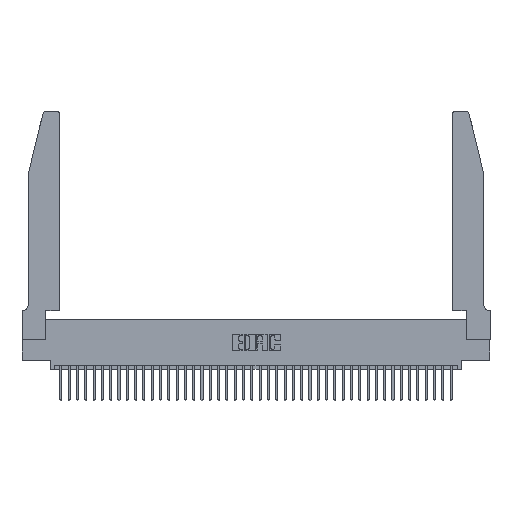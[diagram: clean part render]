
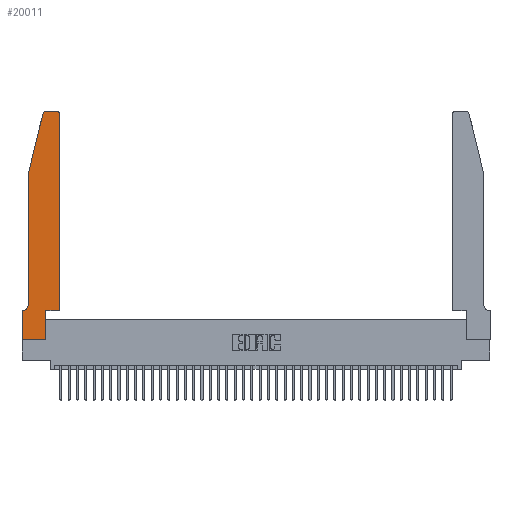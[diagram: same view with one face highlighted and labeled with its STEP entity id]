
A CAD part, top view. The second image highlights one B-rep face of the part: STEP entity #20011.
In plain terms, the highlighted planar face has unit normal (0, 0, 1).
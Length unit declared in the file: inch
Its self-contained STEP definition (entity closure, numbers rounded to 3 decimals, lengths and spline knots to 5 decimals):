
#8 = CARTESIAN_POINT ( 'NONE',  ( 0.0055, 0.42, 0.37 ) ) ;
#233 = VECTOR ( 'NONE', #17555, 39.37008 ) ;
#1323 = CARTESIAN_POINT ( 'NONE',  ( 0.4505, 0.35, 0.37 ) ) ;
#1931 = ORIENTED_EDGE ( 'NONE', *, *, #31756, .T. ) ;
#2160 = EDGE_CURVE ( 'NONE', #39411, #24685, #26172, .T. ) ;
#2168 = VECTOR ( 'NONE', #31009, 39.37008 ) ;
#2701 = VECTOR ( 'NONE', #29917, 39.37008 ) ;
#3124 = DIRECTION ( 'NONE',  ( 1., 0., 0. ) ) ;
#3176 = DIRECTION ( 'NONE',  ( 0., 0., 1. ) ) ;
#3357 = DIRECTION ( 'NONE',  ( -1., 0., 0. ) ) ;
#3690 = VERTEX_POINT ( 'NONE', #20641 ) ;
#3731 = LINE ( 'NONE', #10664, #2701 ) ;
#3998 = ORIENTED_EDGE ( 'NONE', *, *, #31245, .T. ) ;
#4175 = EDGE_CURVE ( 'NONE', #24613, #6546, #34977, .T. ) ;
#4821 = DIRECTION ( 'NONE',  ( 0., -1., 0. ) ) ;
#5491 = CARTESIAN_POINT ( 'NONE',  ( 0.2605, 2.75, 0.37 ) ) ;
#6411 = DIRECTION ( 'NONE',  ( 0., 0., 1. ) ) ;
#6546 = VERTEX_POINT ( 'NONE', #38351 ) ;
#7314 = CARTESIAN_POINT ( 'NONE',  ( 0.25487, 2.72718, 0.37 ) ) ;
#8202 = FACE_OUTER_BOUND ( 'NONE', #25432, .T. ) ;
#8244 = LINE ( 'NONE', #36824, #33868 ) ;
#8453 = VERTEX_POINT ( 'NONE', #12499 ) ;
#8723 = VECTOR ( 'NONE', #19870, 39.37008 ) ;
#10162 = EDGE_CURVE ( 'NONE', #8453, #3690, #25823, .T. ) ;
#10664 = CARTESIAN_POINT ( 'NONE',  ( 0., 0., 0.37 ) ) ;
#11209 = ORIENTED_EDGE ( 'NONE', *, *, #15977, .T. ) ;
#11437 = VECTOR ( 'NONE', #3124, 39.37008 ) ;
#11444 = VERTEX_POINT ( 'NONE', #34825 ) ;
#11750 = ORIENTED_EDGE ( 'NONE', *, *, #10162, .T. ) ;
#12009 = EDGE_CURVE ( 'NONE', #39416, #11444, #35144, .T. ) ;
#12499 = CARTESIAN_POINT ( 'NONE',  ( 0.2865, 0., 0.37 ) ) ;
#12595 = EDGE_CURVE ( 'NONE', #21914, #39416, #13117, .T. ) ;
#13117 = CIRCLE ( 'NONE', #32049, 0.03 ) ;
#13300 = PLANE ( 'NONE',  #21004 ) ;
#14606 = LINE ( 'NONE', #1323, #41025 ) ;
#15320 = ORIENTED_EDGE ( 'NONE', *, *, #22728, .T. ) ;
#15631 = CIRCLE ( 'NONE', #30542, 0.03 ) ;
#15977 = EDGE_CURVE ( 'NONE', #11444, #39411, #15631, .T. ) ;
#16323 = ORIENTED_EDGE ( 'NONE', *, *, #31967, .T. ) ;
#16536 = DIRECTION ( 'NONE',  ( 0., 0., 1. ) ) ;
#16661 = CARTESIAN_POINT ( 'NONE',  ( 0.2865, 0.35, 0.37 ) ) ;
#17555 = DIRECTION ( 'NONE',  ( -0.239, -0.971, 0. ) ) ;
#17736 = DIRECTION ( 'NONE',  ( 0., -1., 0. ) ) ;
#17823 = VERTEX_POINT ( 'NONE', #18836 ) ;
#18129 = CARTESIAN_POINT ( 'NONE',  ( 0.4505, 0.35, 0.37 ) ) ;
#18836 = CARTESIAN_POINT ( 'NONE',  ( 0., 0.35, 0.37 ) ) ;
#19870 = DIRECTION ( 'NONE',  ( 0., 1., 0. ) ) ;
#20011 = ADVANCED_FACE ( 'NONE', ( #8202 ), #13300, .T. ) ;
#20348 = CARTESIAN_POINT ( 'NONE',  ( 0.4205, 2.75, 0.37 ) ) ;
#20420 = CARTESIAN_POINT ( 'NONE',  ( 0.4505, 2.72, 0.37 ) ) ;
#20641 = CARTESIAN_POINT ( 'NONE',  ( 0.2865, 0.35, 0.37 ) ) ;
#21004 = AXIS2_PLACEMENT_3D ( 'NONE', #35638, #16536, #38839 ) ;
#21914 = VERTEX_POINT ( 'NONE', #20420 ) ;
#22636 = CARTESIAN_POINT ( 'NONE',  ( 0., 0., 0.37 ) ) ;
#22663 = CARTESIAN_POINT ( 'NONE',  ( 0.4205, 2.72, 0.37 ) ) ;
#22728 = EDGE_CURVE ( 'NONE', #24685, #24613, #39776, .T. ) ;
#22769 = VERTEX_POINT ( 'NONE', #18129 ) ;
#22851 = DIRECTION ( 'NONE',  ( 0., 0., -1. ) ) ;
#24613 = VERTEX_POINT ( 'NONE', #31008 ) ;
#24685 = VERTEX_POINT ( 'NONE', #41548 ) ;
#25432 = EDGE_LOOP ( 'NONE', ( #26281, #11209, #37771, #15320, #32276, #16323, #26807, #1931, #11750, #28819, #3998, #31803 ) ) ;
#25746 = CARTESIAN_POINT ( 'NONE',  ( 0.284, 2.72, 0.37 ) ) ;
#25823 = LINE ( 'NONE', #16661, #8723 ) ;
#25846 = DIRECTION ( 'NONE',  ( 1., 0., 0. ) ) ;
#26172 = LINE ( 'NONE', #36777, #233 ) ;
#26234 = AXIS2_PLACEMENT_3D ( 'NONE', #8, #22851, #3357 ) ;
#26281 = ORIENTED_EDGE ( 'NONE', *, *, #12009, .T. ) ;
#26807 = ORIENTED_EDGE ( 'NONE', *, *, #28033, .T. ) ;
#27288 = DIRECTION ( 'NONE',  ( 0., 1., 0. ) ) ;
#27509 = LINE ( 'NONE', #38618, #11437 ) ;
#27686 = VECTOR ( 'NONE', #28116, 39.37008 ) ;
#27724 = VERTEX_POINT ( 'NONE', #22636 ) ;
#27794 = CARTESIAN_POINT ( 'NONE',  ( 0.0755, 0.35, 0.37 ) ) ;
#28033 = EDGE_CURVE ( 'NONE', #17823, #27724, #8244, .T. ) ;
#28046 = LINE ( 'NONE', #27794, #2168 ) ;
#28116 = DIRECTION ( 'NONE',  ( -1., 0., 0. ) ) ;
#28819 = ORIENTED_EDGE ( 'NONE', *, *, #32223, .T. ) ;
#28985 = DIRECTION ( 'NONE',  ( 1., 0., 0. ) ) ;
#29917 = DIRECTION ( 'NONE',  ( 1., 0., 0. ) ) ;
#30542 = AXIS2_PLACEMENT_3D ( 'NONE', #25746, #6411, #28985 ) ;
#30686 = CARTESIAN_POINT ( 'NONE',  ( 0.0755, 2., 0.37 ) ) ;
#31008 = CARTESIAN_POINT ( 'NONE',  ( 0.0755, 0.42, 0.37 ) ) ;
#31009 = DIRECTION ( 'NONE',  ( -1., 0., 0. ) ) ;
#31245 = EDGE_CURVE ( 'NONE', #22769, #21914, #14606, .T. ) ;
#31756 = EDGE_CURVE ( 'NONE', #27724, #8453, #3731, .T. ) ;
#31803 = ORIENTED_EDGE ( 'NONE', *, *, #12595, .T. ) ;
#31967 = EDGE_CURVE ( 'NONE', #6546, #17823, #28046, .T. ) ;
#32049 = AXIS2_PLACEMENT_3D ( 'NONE', #22663, #3176, #25846 ) ;
#32223 = EDGE_CURVE ( 'NONE', #3690, #22769, #27509, .T. ) ;
#32276 = ORIENTED_EDGE ( 'NONE', *, *, #4175, .T. ) ;
#33868 = VECTOR ( 'NONE', #17736, 39.37008 ) ;
#34825 = CARTESIAN_POINT ( 'NONE',  ( 0.284, 2.75, 0.37 ) ) ;
#34977 = CIRCLE ( 'NONE', #26234, 0.07 ) ;
#35144 = LINE ( 'NONE', #5491, #27686 ) ;
#35638 = CARTESIAN_POINT ( 'NONE',  ( 0., 0.35, 0.37 ) ) ;
#36777 = CARTESIAN_POINT ( 'NONE',  ( 0.0755, 2., 0.37 ) ) ;
#36824 = CARTESIAN_POINT ( 'NONE',  ( 0., 0., 0.37 ) ) ;
#37771 = ORIENTED_EDGE ( 'NONE', *, *, #2160, .T. ) ;
#37795 = VECTOR ( 'NONE', #4821, 39.37008 ) ;
#38351 = CARTESIAN_POINT ( 'NONE',  ( 0.0055, 0.35, 0.37 ) ) ;
#38618 = CARTESIAN_POINT ( 'NONE',  ( 0.4505, 0.35, 0.37 ) ) ;
#38839 = DIRECTION ( 'NONE',  ( 1., 0., 0. ) ) ;
#39411 = VERTEX_POINT ( 'NONE', #7314 ) ;
#39416 = VERTEX_POINT ( 'NONE', #20348 ) ;
#39776 = LINE ( 'NONE', #30686, #37795 ) ;
#41025 = VECTOR ( 'NONE', #27288, 39.37008 ) ;
#41548 = CARTESIAN_POINT ( 'NONE',  ( 0.0755, 2., 0.37 ) ) ;
